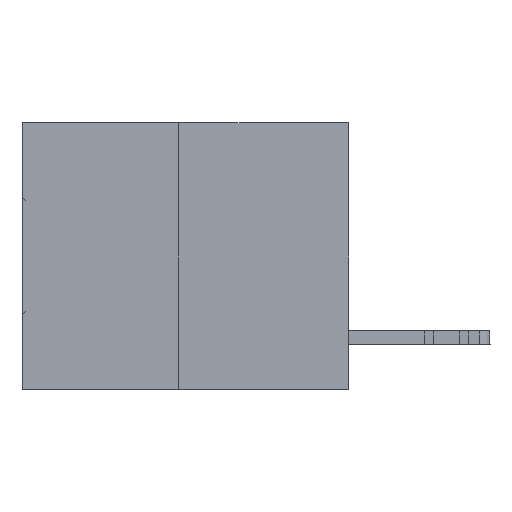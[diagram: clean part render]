
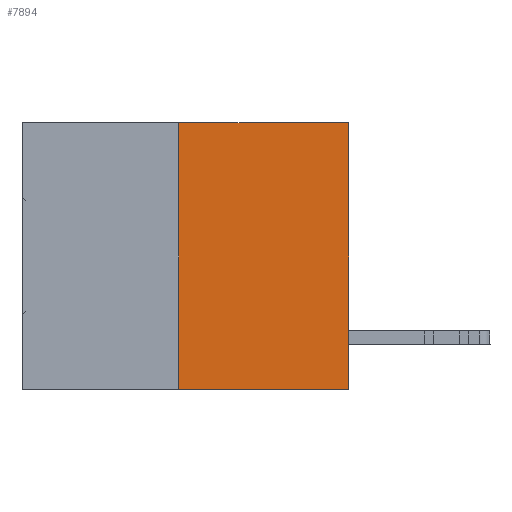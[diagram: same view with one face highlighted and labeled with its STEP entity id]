
A CAD part, left-side view. The second image highlights one B-rep face of the part: STEP entity #7894.
In plain terms, the highlighted planar face has unit normal (-1, 0, 0).
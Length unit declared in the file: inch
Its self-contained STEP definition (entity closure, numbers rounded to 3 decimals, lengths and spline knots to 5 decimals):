
#422 = CARTESIAN_POINT ( 'NONE',  ( 0., 0.6, 0. ) ) ;
#539 = DIRECTION ( 'NONE',  ( 1., 0., 0. ) ) ;
#1971 = FACE_OUTER_BOUND ( 'NONE', #9928, .T. ) ;
#2523 = CARTESIAN_POINT ( 'NONE',  ( 0., 0.6, -0.49 ) ) ;
#2549 = VERTEX_POINT ( 'NONE', #20563 ) ;
#3510 = ORIENTED_EDGE ( 'NONE', *, *, #16363, .T. ) ;
#4645 = VERTEX_POINT ( 'NONE', #9365 ) ;
#5494 = ORIENTED_EDGE ( 'NONE', *, *, #15192, .T. ) ;
#7213 = VECTOR ( 'NONE', #22071, 39.37008 ) ;
#7894 = ADVANCED_FACE ( 'NONE', ( #1971 ), #14147, .F. ) ;
#8284 = CARTESIAN_POINT ( 'NONE',  ( 0., 0., -0.49 ) ) ;
#8679 = VECTOR ( 'NONE', #20866, 39.37008 ) ;
#9365 = CARTESIAN_POINT ( 'NONE',  ( 0., 0.312, 0. ) ) ;
#9928 = EDGE_LOOP ( 'NONE', ( #34770, #3510, #5494, #11105 ) ) ;
#10550 = VECTOR ( 'NONE', #22951, 39.37008 ) ;
#11105 = ORIENTED_EDGE ( 'NONE', *, *, #23413, .F. ) ;
#11221 = DIRECTION ( 'NONE',  ( 0., 0., -1. ) ) ;
#13662 = VERTEX_POINT ( 'NONE', #8284 ) ;
#14147 = PLANE ( 'NONE',  #33674 ) ;
#14500 = LINE ( 'NONE', #28171, #7213 ) ;
#14748 = LINE ( 'NONE', #2523, #8679 ) ;
#15192 = EDGE_CURVE ( 'NONE', #13662, #2549, #30166, .T. ) ;
#15808 = CARTESIAN_POINT ( 'NONE',  ( 0., 0.312, -0.49 ) ) ;
#15938 = VERTEX_POINT ( 'NONE', #15808 ) ;
#16363 = EDGE_CURVE ( 'NONE', #15938, #13662, #14748, .T. ) ;
#18468 = CARTESIAN_POINT ( 'NONE',  ( 0., 0.312, -0.49 ) ) ;
#20111 = CARTESIAN_POINT ( 'NONE',  ( 0., 0., 0. ) ) ;
#20563 = CARTESIAN_POINT ( 'NONE',  ( 0., 0., 0. ) ) ;
#20866 = DIRECTION ( 'NONE',  ( 0., -1., 0. ) ) ;
#22071 = DIRECTION ( 'NONE',  ( 0., -1., 0. ) ) ;
#22951 = DIRECTION ( 'NONE',  ( 0., 0., 1. ) ) ;
#23413 = EDGE_CURVE ( 'NONE', #4645, #2549, #14500, .T. ) ;
#26818 = DIRECTION ( 'NONE',  ( 0., 0., 1. ) ) ;
#27565 = LINE ( 'NONE', #18468, #31514 ) ;
#28046 = EDGE_CURVE ( 'NONE', #15938, #4645, #27565, .T. ) ;
#28171 = CARTESIAN_POINT ( 'NONE',  ( 0., 0.6, 0. ) ) ;
#30166 = LINE ( 'NONE', #20111, #10550 ) ;
#31514 = VECTOR ( 'NONE', #26818, 39.37008 ) ;
#33674 = AXIS2_PLACEMENT_3D ( 'NONE', #422, #539, #11221 ) ;
#34770 = ORIENTED_EDGE ( 'NONE', *, *, #28046, .F. ) ;
